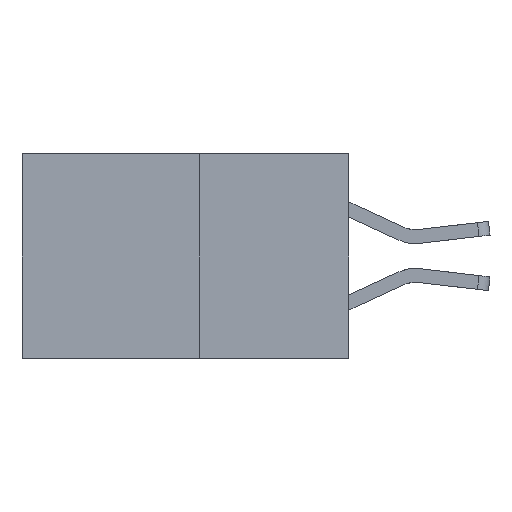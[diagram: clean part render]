
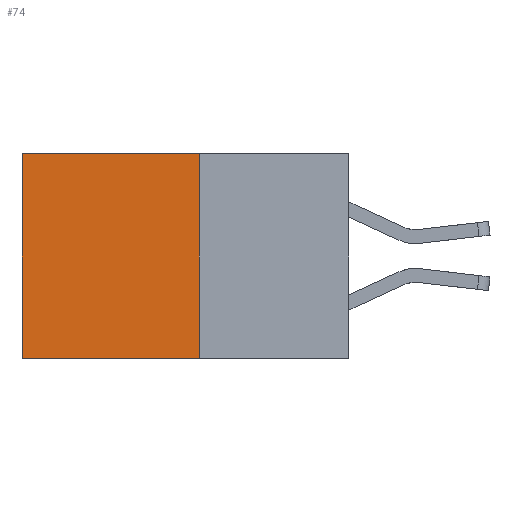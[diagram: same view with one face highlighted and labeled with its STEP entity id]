
A CAD part, left-side view. The second image highlights one B-rep face of the part: STEP entity #74.
In plain terms, the highlighted planar face has unit normal (-1, 0, 0).
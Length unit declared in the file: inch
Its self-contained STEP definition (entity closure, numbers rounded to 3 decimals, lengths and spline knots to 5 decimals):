
#74 = ADVANCED_FACE ( 'NONE', ( #1326 ), #8822, .F. ) ;
#755 = VERTEX_POINT ( 'NONE', #2871 ) ;
#944 = EDGE_LOOP ( 'NONE', ( #3293, #10644, #1660, #3303 ) ) ;
#1028 = DIRECTION ( 'NONE',  ( 0., 0., -1. ) ) ;
#1053 = DIRECTION ( 'NONE',  ( 1., 0., 0. ) ) ;
#1223 = EDGE_CURVE ( 'NONE', #9203, #755, #4935, .T. ) ;
#1326 = FACE_OUTER_BOUND ( 'NONE', #944, .T. ) ;
#1660 = ORIENTED_EDGE ( 'NONE', *, *, #1865, .F. ) ;
#1693 = VERTEX_POINT ( 'NONE', #5069 ) ;
#1865 = EDGE_CURVE ( 'NONE', #9203, #9216, #9930, .T. ) ;
#2224 = DIRECTION ( 'NONE',  ( 0., 0., -1. ) ) ;
#2267 = CARTESIAN_POINT ( 'NONE',  ( 0.277, 0.27, -0.37 ) ) ;
#2564 = CARTESIAN_POINT ( 'NONE',  ( 0.277, 0.27, -0.37 ) ) ;
#2796 = LINE ( 'NONE', #2267, #9255 ) ;
#2871 = CARTESIAN_POINT ( 'NONE',  ( 0.277, 0.59, 0. ) ) ;
#2940 = DIRECTION ( 'NONE',  ( 0., 1., 0. ) ) ;
#3257 = LINE ( 'NONE', #3548, #10119 ) ;
#3293 = ORIENTED_EDGE ( 'NONE', *, *, #8594, .T. ) ;
#3303 = ORIENTED_EDGE ( 'NONE', *, *, #1223, .T. ) ;
#3548 = CARTESIAN_POINT ( 'NONE',  ( 0.277, 0.59, -0.37 ) ) ;
#4935 = LINE ( 'NONE', #9021, #10888 ) ;
#5069 = CARTESIAN_POINT ( 'NONE',  ( 0.277, 0.59, -0.37 ) ) ;
#5099 = DIRECTION ( 'NONE',  ( 0., 0., -1. ) ) ;
#5328 = EDGE_CURVE ( 'NONE', #9216, #1693, #2796, .T. ) ;
#5728 = CARTESIAN_POINT ( 'NONE',  ( 0.277, 0.27, -0.37 ) ) ;
#5760 = CARTESIAN_POINT ( 'NONE',  ( 0.277, 0.27, 0. ) ) ;
#6057 = AXIS2_PLACEMENT_3D ( 'NONE', #8405, #1053, #1028 ) ;
#7562 = VECTOR ( 'NONE', #2224, 39.37008 ) ;
#8405 = CARTESIAN_POINT ( 'NONE',  ( 0.277, 0.27, -0.37 ) ) ;
#8594 = EDGE_CURVE ( 'NONE', #755, #1693, #3257, .T. ) ;
#8822 = PLANE ( 'NONE',  #6057 ) ;
#8851 = DIRECTION ( 'NONE',  ( 0., 1., 0. ) ) ;
#9021 = CARTESIAN_POINT ( 'NONE',  ( 0.277, 0.27, 0. ) ) ;
#9203 = VERTEX_POINT ( 'NONE', #5760 ) ;
#9216 = VERTEX_POINT ( 'NONE', #5728 ) ;
#9255 = VECTOR ( 'NONE', #2940, 39.37008 ) ;
#9930 = LINE ( 'NONE', #2564, #7562 ) ;
#10119 = VECTOR ( 'NONE', #5099, 39.37008 ) ;
#10644 = ORIENTED_EDGE ( 'NONE', *, *, #5328, .F. ) ;
#10888 = VECTOR ( 'NONE', #8851, 39.37008 ) ;
